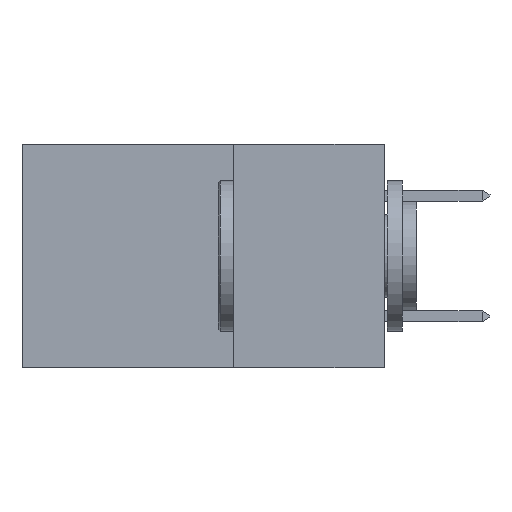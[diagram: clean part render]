
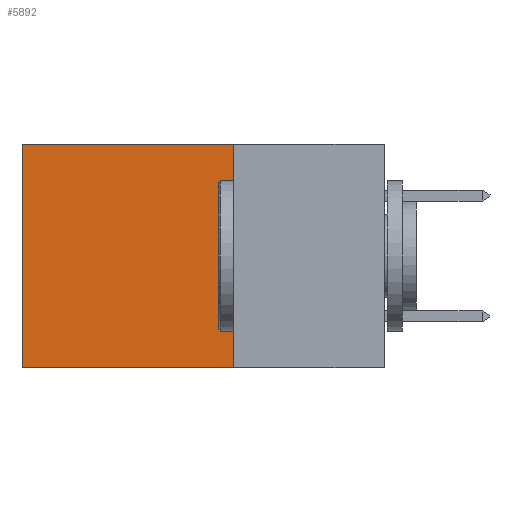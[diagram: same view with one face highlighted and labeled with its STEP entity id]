
A CAD part, left-side view. The second image highlights one B-rep face of the part: STEP entity #5892.
In plain terms, the highlighted planar face has unit normal (-1, 0, 0).
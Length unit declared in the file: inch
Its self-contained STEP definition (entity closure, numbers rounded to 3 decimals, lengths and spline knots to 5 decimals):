
#465 = ORIENTED_EDGE ( 'NONE', *, *, #9492, .F. ) ;
#1102 = VERTEX_POINT ( 'NONE', #14766 ) ;
#5287 = EDGE_CURVE ( 'NONE', #8269, #19446, #11676, .T. ) ;
#5856 = EDGE_CURVE ( 'NONE', #19446, #16737, #12906, .T. ) ;
#5892 = ADVANCED_FACE ( 'NONE', ( #7971 ), #15964, .F. ) ;
#6112 = VECTOR ( 'NONE', #8518, 39.37008 ) ;
#6418 = CARTESIAN_POINT ( 'NONE',  ( 0.2875, 0.25, 0. ) ) ;
#7806 = CARTESIAN_POINT ( 'NONE',  ( 0.2875, 0.6, -0.37 ) ) ;
#7971 = FACE_OUTER_BOUND ( 'NONE', #17782, .T. ) ;
#8189 = ORIENTED_EDGE ( 'NONE', *, *, #5856, .T. ) ;
#8269 = VERTEX_POINT ( 'NONE', #6418 ) ;
#8294 = ORIENTED_EDGE ( 'NONE', *, *, #5287, .T. ) ;
#8493 = VECTOR ( 'NONE', #16774, 39.37008 ) ;
#8518 = DIRECTION ( 'NONE',  ( 0., 1., 0. ) ) ;
#8986 = CARTESIAN_POINT ( 'NONE',  ( 0.2875, 0.25, 0. ) ) ;
#9195 = DIRECTION ( 'NONE',  ( 0., 0., -1. ) ) ;
#9492 = EDGE_CURVE ( 'NONE', #8269, #1102, #15901, .T. ) ;
#11676 = LINE ( 'NONE', #8986, #6112 ) ;
#12906 = LINE ( 'NONE', #16910, #8493 ) ;
#12930 = CARTESIAN_POINT ( 'NONE',  ( 0.2875, 0.6, 0. ) ) ;
#12955 = ORIENTED_EDGE ( 'NONE', *, *, #15981, .F. ) ;
#14766 = CARTESIAN_POINT ( 'NONE',  ( 0.2875, 0.25, -0.37 ) ) ;
#15406 = LINE ( 'NONE', #15737, #19135 ) ;
#15720 = DIRECTION ( 'NONE',  ( 0., 0., -1. ) ) ;
#15737 = CARTESIAN_POINT ( 'NONE',  ( 0.2875, 0.25, -0.37 ) ) ;
#15753 = DIRECTION ( 'NONE',  ( 1., 0., 0. ) ) ;
#15901 = LINE ( 'NONE', #17239, #19630 ) ;
#15964 = PLANE ( 'NONE',  #19450 ) ;
#15981 = EDGE_CURVE ( 'NONE', #1102, #16737, #15406, .T. ) ;
#16006 = CARTESIAN_POINT ( 'NONE',  ( 0.2875, 0.25, 0. ) ) ;
#16737 = VERTEX_POINT ( 'NONE', #7806 ) ;
#16774 = DIRECTION ( 'NONE',  ( 0., 0., -1. ) ) ;
#16910 = CARTESIAN_POINT ( 'NONE',  ( 0.2875, 0.6, 0. ) ) ;
#17239 = CARTESIAN_POINT ( 'NONE',  ( 0.2875, 0.25, 0. ) ) ;
#17321 = DIRECTION ( 'NONE',  ( 0., 1., 0. ) ) ;
#17782 = EDGE_LOOP ( 'NONE', ( #8189, #12955, #465, #8294 ) ) ;
#19135 = VECTOR ( 'NONE', #17321, 39.37008 ) ;
#19446 = VERTEX_POINT ( 'NONE', #12930 ) ;
#19450 = AXIS2_PLACEMENT_3D ( 'NONE', #16006, #15753, #15720 ) ;
#19630 = VECTOR ( 'NONE', #9195, 39.37008 ) ;
